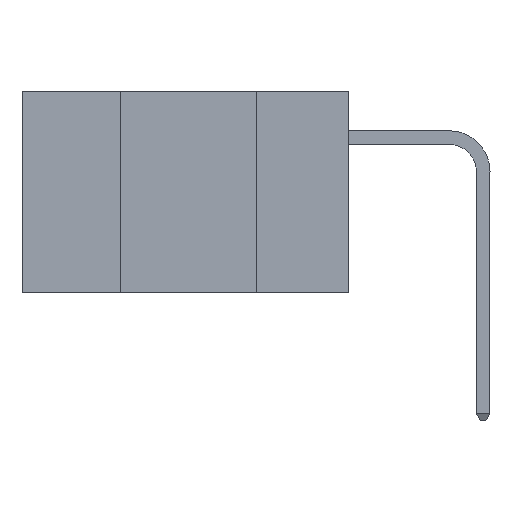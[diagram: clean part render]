
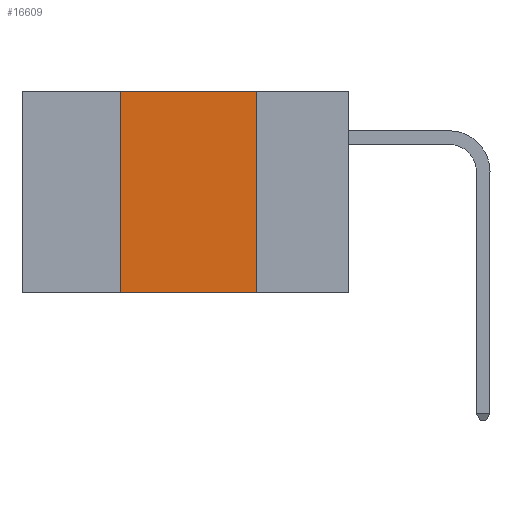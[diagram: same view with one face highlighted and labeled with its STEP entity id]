
A CAD part, left-side view. The second image highlights one B-rep face of the part: STEP entity #16609.
In plain terms, the highlighted planar face has unit normal (-1, 0, 0).
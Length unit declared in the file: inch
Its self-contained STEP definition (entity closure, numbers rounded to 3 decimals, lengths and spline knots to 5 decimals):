
#153 = LINE ( 'NONE', #2622, #17140 ) ;
#162 = LINE ( 'NONE', #20240, #17685 ) ;
#242 = CARTESIAN_POINT ( 'NONE',  ( 0., 0.42, 0. ) ) ;
#864 = EDGE_CURVE ( 'NONE', #11333, #4874, #153, .T. ) ;
#1171 = VERTEX_POINT ( 'NONE', #16583 ) ;
#2622 = CARTESIAN_POINT ( 'NONE',  ( 0., 0.6, -0.37 ) ) ;
#2867 = EDGE_CURVE ( 'NONE', #3810, #1171, #5968, .T. ) ;
#3049 = ORIENTED_EDGE ( 'NONE', *, *, #2867, .F. ) ;
#3296 = DIRECTION ( 'NONE',  ( 0., 0., 1. ) ) ;
#3510 = CARTESIAN_POINT ( 'NONE',  ( 0., 0.42, -0.37 ) ) ;
#3686 = VECTOR ( 'NONE', #19661, 39.37008 ) ;
#3810 = VERTEX_POINT ( 'NONE', #242 ) ;
#4874 = VERTEX_POINT ( 'NONE', #16514 ) ;
#4931 = DIRECTION ( 'NONE',  ( 1., 0., 0. ) ) ;
#5968 = LINE ( 'NONE', #18005, #3686 ) ;
#6260 = ORIENTED_EDGE ( 'NONE', *, *, #864, .T. ) ;
#7310 = EDGE_LOOP ( 'NONE', ( #19671, #3049, #9734, #6260 ) ) ;
#7586 = DIRECTION ( 'NONE',  ( 0., -1., 0. ) ) ;
#8125 = DIRECTION ( 'NONE',  ( 0., 0., -1. ) ) ;
#9262 = EDGE_CURVE ( 'NONE', #1171, #4874, #162, .T. ) ;
#9734 = ORIENTED_EDGE ( 'NONE', *, *, #20081, .F. ) ;
#9870 = CARTESIAN_POINT ( 'NONE',  ( 0., 0.6, 0. ) ) ;
#11333 = VERTEX_POINT ( 'NONE', #3510 ) ;
#11891 = AXIS2_PLACEMENT_3D ( 'NONE', #9870, #4931, #8125 ) ;
#14145 = FACE_OUTER_BOUND ( 'NONE', #7310, .T. ) ;
#15234 = VECTOR ( 'NONE', #3296, 39.37008 ) ;
#15378 = DIRECTION ( 'NONE',  ( 0., 0., -1. ) ) ;
#16464 = CARTESIAN_POINT ( 'NONE',  ( 0., 0.42, 0. ) ) ;
#16514 = CARTESIAN_POINT ( 'NONE',  ( 0., 0.17, -0.37 ) ) ;
#16583 = CARTESIAN_POINT ( 'NONE',  ( 0., 0.17, 0. ) ) ;
#16609 = ADVANCED_FACE ( 'NONE', ( #14145 ), #19577, .F. ) ;
#17140 = VECTOR ( 'NONE', #7586, 39.37008 ) ;
#17685 = VECTOR ( 'NONE', #15378, 39.37008 ) ;
#18005 = CARTESIAN_POINT ( 'NONE',  ( 0., 0.6, 0. ) ) ;
#19577 = PLANE ( 'NONE',  #11891 ) ;
#19661 = DIRECTION ( 'NONE',  ( 0., -1., 0. ) ) ;
#19671 = ORIENTED_EDGE ( 'NONE', *, *, #9262, .F. ) ;
#20081 = EDGE_CURVE ( 'NONE', #11333, #3810, #20877, .T. ) ;
#20240 = CARTESIAN_POINT ( 'NONE',  ( 0., 0.17, 0. ) ) ;
#20877 = LINE ( 'NONE', #16464, #15234 ) ;
